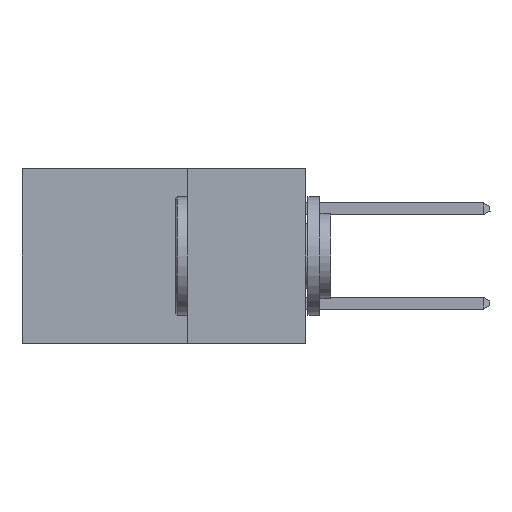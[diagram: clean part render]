
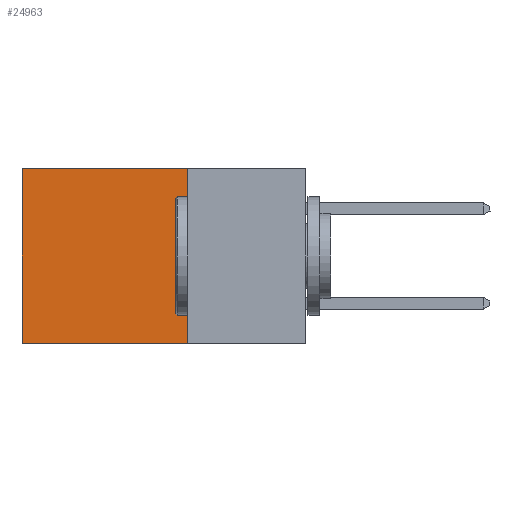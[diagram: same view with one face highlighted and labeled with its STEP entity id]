
A CAD part, left-side view. The second image highlights one B-rep face of the part: STEP entity #24963.
In plain terms, the highlighted planar face has unit normal (-1, 0, 0).
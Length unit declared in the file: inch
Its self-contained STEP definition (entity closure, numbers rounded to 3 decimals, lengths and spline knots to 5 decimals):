
#1518 = DIRECTION ( 'NONE',  ( 0., 1., 0. ) ) ;
#2199 = ORIENTED_EDGE ( 'NONE', *, *, #26746, .T. ) ;
#2975 = PLANE ( 'NONE',  #21306 ) ;
#3082 = DIRECTION ( 'NONE',  ( 0., 0., -1. ) ) ;
#3657 = CARTESIAN_POINT ( 'NONE',  ( 0.298, 0.6, 0. ) ) ;
#4147 = CARTESIAN_POINT ( 'NONE',  ( 0.298, 0.25, 0. ) ) ;
#4329 = LINE ( 'NONE', #30169, #12610 ) ;
#4349 = DIRECTION ( 'NONE',  ( 0., 1., 0. ) ) ;
#4648 = VECTOR ( 'NONE', #15014, 39.37008 ) ;
#4882 = FACE_OUTER_BOUND ( 'NONE', #13218, .T. ) ;
#7710 = VECTOR ( 'NONE', #4349, 39.37008 ) ;
#7813 = CARTESIAN_POINT ( 'NONE',  ( 0.298, 0.25, 0. ) ) ;
#8462 = EDGE_CURVE ( 'NONE', #11407, #10635, #27254, .T. ) ;
#8950 = CARTESIAN_POINT ( 'NONE',  ( 0.298, 0.25, -0.37 ) ) ;
#8984 = VECTOR ( 'NONE', #29834, 39.37008 ) ;
#10460 = CARTESIAN_POINT ( 'NONE',  ( 0.298, 0.25, 0. ) ) ;
#10635 = VERTEX_POINT ( 'NONE', #8950 ) ;
#10650 = CARTESIAN_POINT ( 'NONE',  ( 0.298, 0.6, -0.37 ) ) ;
#11407 = VERTEX_POINT ( 'NONE', #28424 ) ;
#11598 = LINE ( 'NONE', #3657, #8984 ) ;
#12610 = VECTOR ( 'NONE', #1518, 39.37008 ) ;
#13218 = EDGE_LOOP ( 'NONE', ( #18585, #18454, #17235, #2199 ) ) ;
#13931 = EDGE_CURVE ( 'NONE', #29558, #20865, #11598, .T. ) ;
#15014 = DIRECTION ( 'NONE',  ( 0., 0., -1. ) ) ;
#15650 = CARTESIAN_POINT ( 'NONE',  ( 0.298, 0.6, 0. ) ) ;
#17235 = ORIENTED_EDGE ( 'NONE', *, *, #8462, .F. ) ;
#18454 = ORIENTED_EDGE ( 'NONE', *, *, #22008, .F. ) ;
#18585 = ORIENTED_EDGE ( 'NONE', *, *, #13931, .T. ) ;
#19964 = DIRECTION ( 'NONE',  ( 1., 0., 0. ) ) ;
#20865 = VERTEX_POINT ( 'NONE', #10650 ) ;
#21306 = AXIS2_PLACEMENT_3D ( 'NONE', #10460, #19964, #3082 ) ;
#21678 = LINE ( 'NONE', #4147, #7710 ) ;
#22008 = EDGE_CURVE ( 'NONE', #10635, #20865, #4329, .T. ) ;
#24963 = ADVANCED_FACE ( 'NONE', ( #4882 ), #2975, .F. ) ;
#26746 = EDGE_CURVE ( 'NONE', #11407, #29558, #21678, .T. ) ;
#27254 = LINE ( 'NONE', #7813, #4648 ) ;
#28424 = CARTESIAN_POINT ( 'NONE',  ( 0.298, 0.25, 0. ) ) ;
#29558 = VERTEX_POINT ( 'NONE', #15650 ) ;
#29834 = DIRECTION ( 'NONE',  ( 0., 0., -1. ) ) ;
#30169 = CARTESIAN_POINT ( 'NONE',  ( 0.298, 0.25, -0.37 ) ) ;
